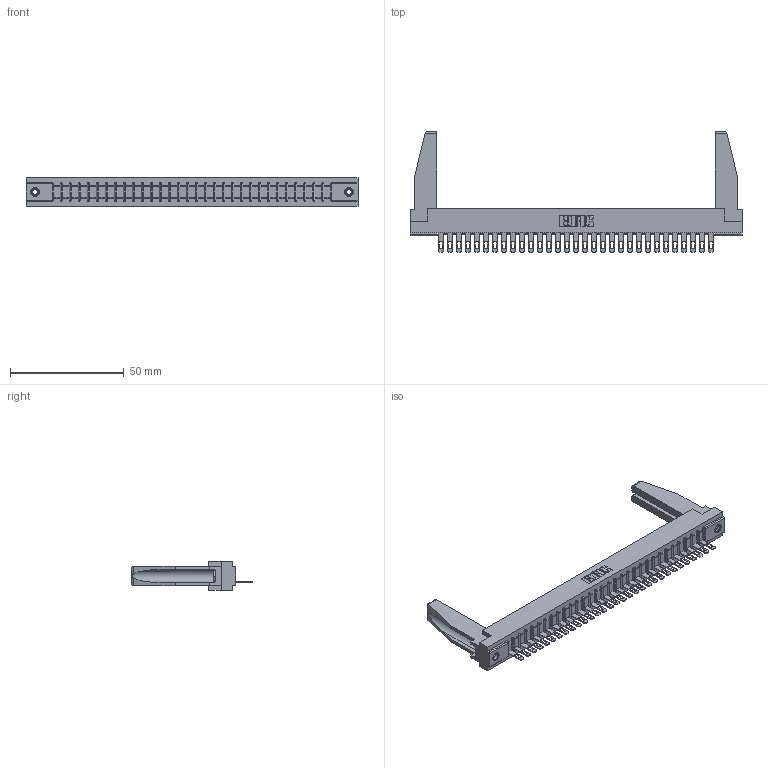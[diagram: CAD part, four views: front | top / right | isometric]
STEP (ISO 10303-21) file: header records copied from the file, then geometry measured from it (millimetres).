
FILE_DESCRIPTION (( 'STEP AP203' ), '1' );
FILE_NAME ('307-031-405-178.STEP', '2020-09-28T12:37:35', ( '' ), ( '' ), 'SwSTEP 2.0', 'SolidWorks 2020', '' );
FILE_SCHEMA (( 'CONFIG_CONTROL_DESIGN' ));
Length unit declared in the file: inch
Products named in the file (5): 307-220-078; 345-250-001_345-250-001-102; 307 Part_.156 Dia Mounting Holes; 307-031-405-178; 307-290-001_505
Assembly tree (36 placements, depth 2):
  307-031-405-178
    307 Part_.156 Dia Mounting Holes
    307-290-001_505  x31
    307-220-078  x2
    345-250-001_345-250-001-102  x2
Bounding box: 145.85 x 52.88 x 12.7 mm (x, y, z)
Volume: 19113.3 mm3; surface area: 19972.4 mm2
Topology: 36 solids, 36 shells, 2016 faces, 5675 edges, 3646 vertices
Faces by surface type: plane 1270, cylinder 666, sphere 64, cone 12, torus 4
Entity records: 30345 total; most frequent: CARTESIAN_POINT 5106, ORIENTED_EDGE 5048, DIRECTION 4930, EDGE_CURVE 2524, VECTOR 1934, LINE 1934, VERTEX_POINT 1632, AXIS2_PLACEMENT_3D 1498
